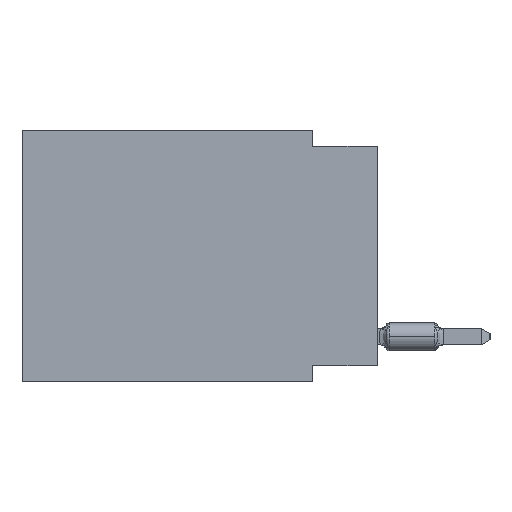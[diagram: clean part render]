
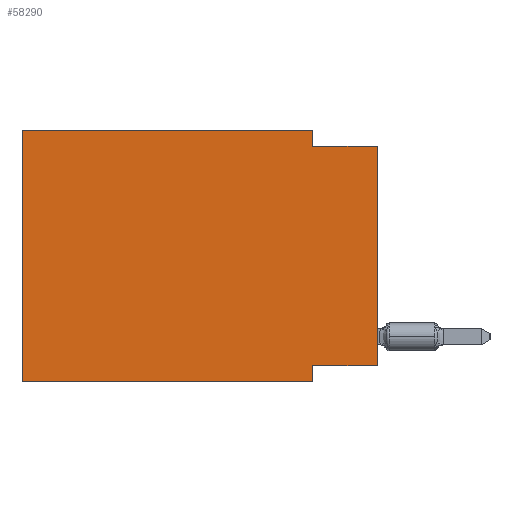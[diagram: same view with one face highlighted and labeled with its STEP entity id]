
A CAD part, left-side view. The second image highlights one B-rep face of the part: STEP entity #58290.
In plain terms, the highlighted planar face has unit normal (-1, 0, 0).
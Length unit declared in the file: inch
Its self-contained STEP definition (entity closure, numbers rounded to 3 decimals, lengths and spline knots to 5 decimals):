
#988 = ORIENTED_EDGE ( 'NONE', *, *, #50872, .F. ) ;
#3262 = VECTOR ( 'NONE', #50020, 39.37008 ) ;
#4306 = CARTESIAN_POINT ( 'NONE',  ( 0., 0., -0.365 ) ) ;
#7468 = VERTEX_POINT ( 'NONE', #71227 ) ;
#7819 = DIRECTION ( 'NONE',  ( 0., 0., -1. ) ) ;
#9701 = LINE ( 'NONE', #56606, #3262 ) ;
#9800 = LINE ( 'NONE', #76902, #41863 ) ;
#11570 = ORIENTED_EDGE ( 'NONE', *, *, #42922, .F. ) ;
#12069 = CARTESIAN_POINT ( 'NONE',  ( 0., 0.55, -0.39 ) ) ;
#14138 = VERTEX_POINT ( 'NONE', #64155 ) ;
#15254 = PLANE ( 'NONE',  #27711 ) ;
#16163 = LINE ( 'NONE', #49923, #60198 ) ;
#17023 = DIRECTION ( 'NONE',  ( 0., 0., 1. ) ) ;
#18611 = VERTEX_POINT ( 'NONE', #31310 ) ;
#19281 = CARTESIAN_POINT ( 'NONE',  ( 0., 0.55, 0. ) ) ;
#19604 = LINE ( 'NONE', #67407, #73617 ) ;
#20582 = VECTOR ( 'NONE', #76155, 39.37008 ) ;
#21631 = VERTEX_POINT ( 'NONE', #32928 ) ;
#24426 = CARTESIAN_POINT ( 'NONE',  ( 0., 0., -0.365 ) ) ;
#25787 = EDGE_CURVE ( 'NONE', #49652, #70509, #16163, .T. ) ;
#26296 = ORIENTED_EDGE ( 'NONE', *, *, #55487, .F. ) ;
#27711 = AXIS2_PLACEMENT_3D ( 'NONE', #28839, #81091, #7819 ) ;
#28839 = CARTESIAN_POINT ( 'NONE',  ( 0., 0.55, 0. ) ) ;
#29029 = EDGE_CURVE ( 'NONE', #14138, #56463, #39210, .T. ) ;
#29880 = CARTESIAN_POINT ( 'NONE',  ( 0., 0., -0.025 ) ) ;
#31310 = CARTESIAN_POINT ( 'NONE',  ( 0., 0.1, -0.365 ) ) ;
#31793 = DIRECTION ( 'NONE',  ( 0., -1., 0. ) ) ;
#32928 = CARTESIAN_POINT ( 'NONE',  ( 0., 0.1, -0.025 ) ) ;
#39049 = CARTESIAN_POINT ( 'NONE',  ( 0., 0.1, -0.39 ) ) ;
#39210 = LINE ( 'NONE', #12069, #40892 ) ;
#40892 = VECTOR ( 'NONE', #31793, 39.37008 ) ;
#41863 = VECTOR ( 'NONE', #50117, 39.37008 ) ;
#42289 = ORIENTED_EDGE ( 'NONE', *, *, #25787, .T. ) ;
#42922 = EDGE_CURVE ( 'NONE', #21631, #70509, #9800, .T. ) ;
#43555 = ORIENTED_EDGE ( 'NONE', *, *, #55669, .F. ) ;
#49179 = DIRECTION ( 'NONE',  ( 0., 0., -1. ) ) ;
#49652 = VERTEX_POINT ( 'NONE', #4306 ) ;
#49923 = CARTESIAN_POINT ( 'NONE',  ( 0., 0., 0. ) ) ;
#50020 = DIRECTION ( 'NONE',  ( 0., 0., -1. ) ) ;
#50117 = DIRECTION ( 'NONE',  ( 0., -1., 0. ) ) ;
#50872 = EDGE_CURVE ( 'NONE', #7468, #21631, #9701, .T. ) ;
#51974 = EDGE_CURVE ( 'NONE', #18611, #56463, #82972, .T. ) ;
#54736 = FACE_OUTER_BOUND ( 'NONE', #70530, .T. ) ;
#55487 = EDGE_CURVE ( 'NONE', #14138, #84234, #19604, .T. ) ;
#55669 = EDGE_CURVE ( 'NONE', #84234, #7468, #69124, .T. ) ;
#56463 = VERTEX_POINT ( 'NONE', #39049 ) ;
#56606 = CARTESIAN_POINT ( 'NONE',  ( 0., 0.1, 0. ) ) ;
#57176 = EDGE_CURVE ( 'NONE', #49652, #18611, #77515, .T. ) ;
#58290 = ADVANCED_FACE ( 'NONE', ( #54736 ), #15254, .F. ) ;
#60198 = VECTOR ( 'NONE', #17023, 39.37008 ) ;
#60387 = DIRECTION ( 'NONE',  ( 0., 0., 1. ) ) ;
#62345 = CARTESIAN_POINT ( 'NONE',  ( 0., 0.1, -0.39 ) ) ;
#64155 = CARTESIAN_POINT ( 'NONE',  ( 0., 0.55, -0.39 ) ) ;
#66782 = VECTOR ( 'NONE', #84094, 39.37008 ) ;
#67407 = CARTESIAN_POINT ( 'NONE',  ( 0., 0.55, 0. ) ) ;
#69124 = LINE ( 'NONE', #82746, #20582 ) ;
#69779 = ORIENTED_EDGE ( 'NONE', *, *, #29029, .T. ) ;
#70509 = VERTEX_POINT ( 'NONE', #29880 ) ;
#70530 = EDGE_LOOP ( 'NONE', ( #42289, #11570, #988, #43555, #26296, #69779, #71474, #79991 ) ) ;
#71227 = CARTESIAN_POINT ( 'NONE',  ( 0., 0.1, 0. ) ) ;
#71474 = ORIENTED_EDGE ( 'NONE', *, *, #51974, .F. ) ;
#73432 = VECTOR ( 'NONE', #49179, 39.37008 ) ;
#73617 = VECTOR ( 'NONE', #60387, 39.37008 ) ;
#76155 = DIRECTION ( 'NONE',  ( 0., -1., 0. ) ) ;
#76902 = CARTESIAN_POINT ( 'NONE',  ( 0., 0., -0.025 ) ) ;
#77515 = LINE ( 'NONE', #24426, #66782 ) ;
#79991 = ORIENTED_EDGE ( 'NONE', *, *, #57176, .F. ) ;
#81091 = DIRECTION ( 'NONE',  ( 1., 0., 0. ) ) ;
#82746 = CARTESIAN_POINT ( 'NONE',  ( 0., 0.55, 0. ) ) ;
#82972 = LINE ( 'NONE', #62345, #73432 ) ;
#84094 = DIRECTION ( 'NONE',  ( 0., 1., 0. ) ) ;
#84234 = VERTEX_POINT ( 'NONE', #19281 ) ;
